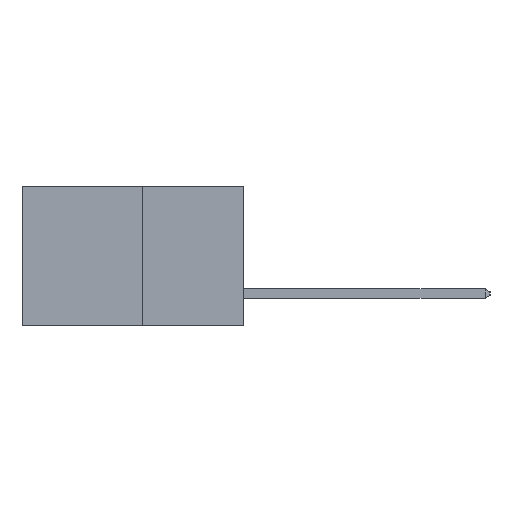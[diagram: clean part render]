
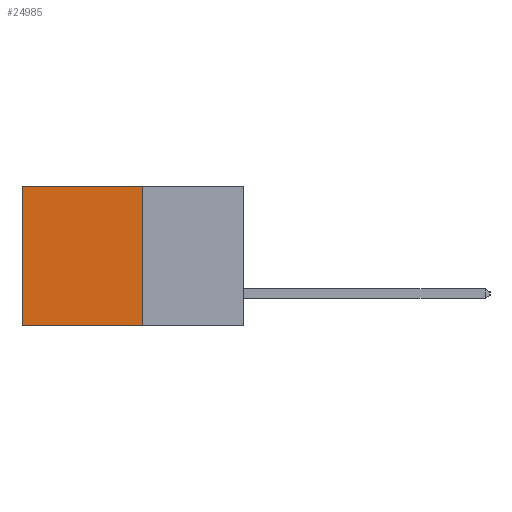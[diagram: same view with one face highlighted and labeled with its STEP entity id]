
A CAD part, left-side view. The second image highlights one B-rep face of the part: STEP entity #24985.
In plain terms, the highlighted planar face has unit normal (-1, 0, 0).
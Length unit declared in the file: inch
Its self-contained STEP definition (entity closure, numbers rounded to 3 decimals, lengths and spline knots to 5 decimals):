
#684 = LINE ( 'NONE', #15811, #3591 ) ;
#1390 = EDGE_CURVE ( 'NONE', #23954, #8872, #9611, .T. ) ;
#2005 = DIRECTION ( 'NONE',  ( 0., 1., 0. ) ) ;
#2353 = ORIENTED_EDGE ( 'NONE', *, *, #11811, .F. ) ;
#2436 = DIRECTION ( 'NONE',  ( 1., 0., 0. ) ) ;
#3591 = VECTOR ( 'NONE', #2005, 39.37008 ) ;
#4222 = CARTESIAN_POINT ( 'NONE',  ( 0.277, 0.59, -0.37 ) ) ;
#4681 = DIRECTION ( 'NONE',  ( 0., 0., -1. ) ) ;
#6187 = CARTESIAN_POINT ( 'NONE',  ( 0.277, 0.27, 0. ) ) ;
#6249 = VECTOR ( 'NONE', #4681, 39.37008 ) ;
#8131 = DIRECTION ( 'NONE',  ( 0., 1., 0. ) ) ;
#8461 = FACE_OUTER_BOUND ( 'NONE', #15649, .T. ) ;
#8684 = CARTESIAN_POINT ( 'NONE',  ( 0.277, 0.27, -0.37 ) ) ;
#8872 = VERTEX_POINT ( 'NONE', #23286 ) ;
#9188 = EDGE_CURVE ( 'NONE', #23954, #17055, #17420, .T. ) ;
#9542 = DIRECTION ( 'NONE',  ( 0., 0., -1. ) ) ;
#9611 = LINE ( 'NONE', #19674, #23951 ) ;
#10369 = PLANE ( 'NONE',  #18724 ) ;
#10808 = ORIENTED_EDGE ( 'NONE', *, *, #9188, .F. ) ;
#10836 = CARTESIAN_POINT ( 'NONE',  ( 0.277, 0.27, -0.37 ) ) ;
#11445 = CARTESIAN_POINT ( 'NONE',  ( 0.277, 0.59, -0.37 ) ) ;
#11811 = EDGE_CURVE ( 'NONE', #17055, #20082, #684, .T. ) ;
#14375 = CARTESIAN_POINT ( 'NONE',  ( 0.277, 0.27, -0.37 ) ) ;
#15224 = VECTOR ( 'NONE', #9542, 39.37008 ) ;
#15649 = EDGE_LOOP ( 'NONE', ( #25099, #2353, #10808, #23917 ) ) ;
#15811 = CARTESIAN_POINT ( 'NONE',  ( 0.277, 0.27, -0.37 ) ) ;
#16371 = DIRECTION ( 'NONE',  ( 0., 0., -1. ) ) ;
#17055 = VERTEX_POINT ( 'NONE', #10836 ) ;
#17420 = LINE ( 'NONE', #8684, #6249 ) ;
#18724 = AXIS2_PLACEMENT_3D ( 'NONE', #14375, #2436, #16371 ) ;
#19060 = EDGE_CURVE ( 'NONE', #8872, #20082, #20352, .T. ) ;
#19674 = CARTESIAN_POINT ( 'NONE',  ( 0.277, 0.27, 0. ) ) ;
#20082 = VERTEX_POINT ( 'NONE', #4222 ) ;
#20352 = LINE ( 'NONE', #11445, #15224 ) ;
#23286 = CARTESIAN_POINT ( 'NONE',  ( 0.277, 0.59, 0. ) ) ;
#23917 = ORIENTED_EDGE ( 'NONE', *, *, #1390, .T. ) ;
#23951 = VECTOR ( 'NONE', #8131, 39.37008 ) ;
#23954 = VERTEX_POINT ( 'NONE', #6187 ) ;
#24985 = ADVANCED_FACE ( 'NONE', ( #8461 ), #10369, .F. ) ;
#25099 = ORIENTED_EDGE ( 'NONE', *, *, #19060, .T. ) ;
